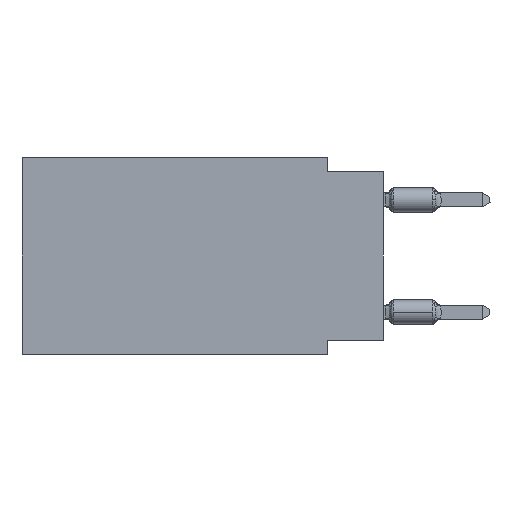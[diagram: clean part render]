
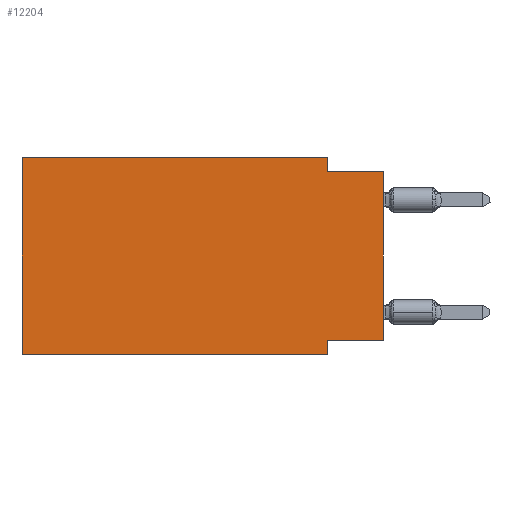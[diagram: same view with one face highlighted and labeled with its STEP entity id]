
A CAD part, left-side view. The second image highlights one B-rep face of the part: STEP entity #12204.
In plain terms, the highlighted planar face has unit normal (-1, 0, 0).
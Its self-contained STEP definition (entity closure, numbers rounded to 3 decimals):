
#708 = ORIENTED_EDGE ( 'NONE', *, *, #18499, .T. ) ;
#780 = VECTOR ( 'NONE', #13681, 1000. ) ;
#789 = LINE ( 'NONE', #4292, #7676 ) ;
#897 = CARTESIAN_POINT ( 'NONE',  ( 0., 2.54, -8.89 ) ) ;
#940 = DIRECTION ( 'NONE',  ( 0., 1., 0. ) ) ;
#1457 = EDGE_LOOP ( 'NONE', ( #708, #12259, #9450, #11400, #1572, #5648, #8041, #4074 ) ) ;
#1572 = ORIENTED_EDGE ( 'NONE', *, *, #16469, .F. ) ;
#2459 = VERTEX_POINT ( 'NONE', #5473 ) ;
#2463 = CARTESIAN_POINT ( 'NONE',  ( 0., 16.383, 0. ) ) ;
#2924 = DIRECTION ( 'NONE',  ( 0., -1., 0. ) ) ;
#3069 = VERTEX_POINT ( 'NONE', #3420 ) ;
#3372 = FACE_OUTER_BOUND ( 'NONE', #1457, .T. ) ;
#3420 = CARTESIAN_POINT ( 'NONE',  ( 0., 2.54, -8.255 ) ) ;
#4074 = ORIENTED_EDGE ( 'NONE', *, *, #22997, .F. ) ;
#4217 = EDGE_CURVE ( 'NONE', #3069, #10695, #9323, .T. ) ;
#4292 = CARTESIAN_POINT ( 'NONE',  ( 0., 0., 0. ) ) ;
#4757 = VERTEX_POINT ( 'NONE', #6420 ) ;
#5030 = CARTESIAN_POINT ( 'NONE',  ( 0., 16.383, 0. ) ) ;
#5082 = CARTESIAN_POINT ( 'NONE',  ( 0., 16.383, -8.89 ) ) ;
#5473 = CARTESIAN_POINT ( 'NONE',  ( 0., 0., -8.255 ) ) ;
#5648 = ORIENTED_EDGE ( 'NONE', *, *, #6364, .T. ) ;
#5852 = DIRECTION ( 'NONE',  ( 0., -1., 0. ) ) ;
#5985 = LINE ( 'NONE', #2463, #11951 ) ;
#6214 = CARTESIAN_POINT ( 'NONE',  ( 0., 0., -8.255 ) ) ;
#6364 = EDGE_CURVE ( 'NONE', #8123, #10695, #21096, .T. ) ;
#6420 = CARTESIAN_POINT ( 'NONE',  ( 0., 2.54, 0. ) ) ;
#7108 = VERTEX_POINT ( 'NONE', #10297 ) ;
#7676 = VECTOR ( 'NONE', #17026, 1000. ) ;
#8041 = ORIENTED_EDGE ( 'NONE', *, *, #4217, .F. ) ;
#8123 = VERTEX_POINT ( 'NONE', #21430 ) ;
#8334 = VECTOR ( 'NONE', #12215, 1000. ) ;
#8740 = PLANE ( 'NONE',  #23088 ) ;
#9215 = VERTEX_POINT ( 'NONE', #15282 ) ;
#9323 = LINE ( 'NONE', #21935, #12639 ) ;
#9450 = ORIENTED_EDGE ( 'NONE', *, *, #18095, .F. ) ;
#10213 = EDGE_CURVE ( 'NONE', #17060, #7108, #10868, .T. ) ;
#10297 = CARTESIAN_POINT ( 'NONE',  ( 0., 0., -0.635 ) ) ;
#10621 = LINE ( 'NONE', #5030, #780 ) ;
#10695 = VERTEX_POINT ( 'NONE', #897 ) ;
#10868 = LINE ( 'NONE', #17999, #18132 ) ;
#11057 = DIRECTION ( 'NONE',  ( 0., 0., -1. ) ) ;
#11182 = VECTOR ( 'NONE', #17291, 1000. ) ;
#11400 = ORIENTED_EDGE ( 'NONE', *, *, #13355, .F. ) ;
#11794 = DIRECTION ( 'NONE',  ( 0., 0., -1. ) ) ;
#11951 = VECTOR ( 'NONE', #2924, 1000. ) ;
#12204 = ADVANCED_FACE ( 'NONE', ( #3372 ), #8740, .F. ) ;
#12215 = DIRECTION ( 'NONE',  ( 0., -1., 0. ) ) ;
#12259 = ORIENTED_EDGE ( 'NONE', *, *, #10213, .F. ) ;
#12639 = VECTOR ( 'NONE', #11057, 1000. ) ;
#12788 = CARTESIAN_POINT ( 'NONE',  ( 0., 2.54, -0.635 ) ) ;
#13355 = EDGE_CURVE ( 'NONE', #9215, #4757, #5985, .T. ) ;
#13681 = DIRECTION ( 'NONE',  ( 0., 0., 1. ) ) ;
#13770 = LINE ( 'NONE', #22879, #11182 ) ;
#15282 = CARTESIAN_POINT ( 'NONE',  ( 0., 16.383, 0. ) ) ;
#15306 = VECTOR ( 'NONE', #940, 1000. ) ;
#15405 = DIRECTION ( 'NONE',  ( 1., 0., 0. ) ) ;
#16469 = EDGE_CURVE ( 'NONE', #8123, #9215, #10621, .T. ) ;
#17026 = DIRECTION ( 'NONE',  ( 0., 0., 1. ) ) ;
#17060 = VERTEX_POINT ( 'NONE', #12788 ) ;
#17184 = CARTESIAN_POINT ( 'NONE',  ( 0., 16.383, 0. ) ) ;
#17291 = DIRECTION ( 'NONE',  ( 0., 0., -1. ) ) ;
#17419 = LINE ( 'NONE', #6214, #15306 ) ;
#17999 = CARTESIAN_POINT ( 'NONE',  ( 0., 0., -0.635 ) ) ;
#18095 = EDGE_CURVE ( 'NONE', #4757, #17060, #13770, .T. ) ;
#18132 = VECTOR ( 'NONE', #5852, 1000. ) ;
#18499 = EDGE_CURVE ( 'NONE', #2459, #7108, #789, .T. ) ;
#21096 = LINE ( 'NONE', #5082, #8334 ) ;
#21430 = CARTESIAN_POINT ( 'NONE',  ( 0., 16.383, -8.89 ) ) ;
#21935 = CARTESIAN_POINT ( 'NONE',  ( 0., 2.54, -8.89 ) ) ;
#22879 = CARTESIAN_POINT ( 'NONE',  ( 0., 2.54, 0. ) ) ;
#22997 = EDGE_CURVE ( 'NONE', #2459, #3069, #17419, .T. ) ;
#23088 = AXIS2_PLACEMENT_3D ( 'NONE', #17184, #15405, #11794 ) ;
